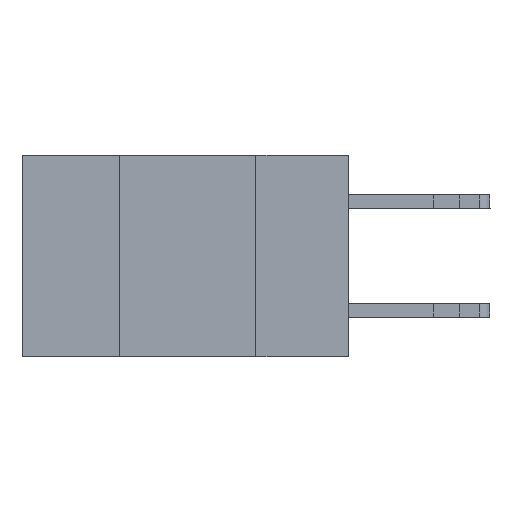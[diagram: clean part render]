
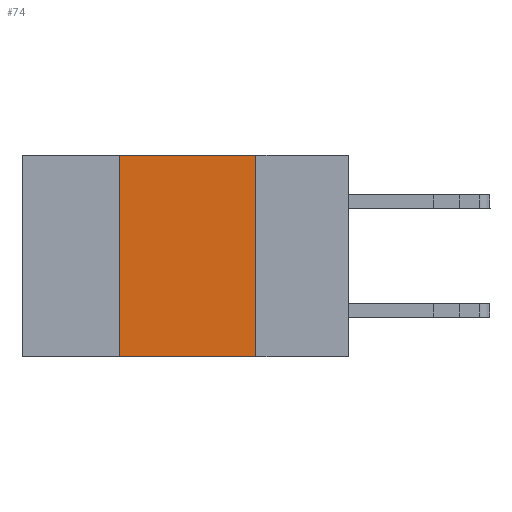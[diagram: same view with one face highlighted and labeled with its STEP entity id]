
A CAD part, left-side view. The second image highlights one B-rep face of the part: STEP entity #74.
In plain terms, the highlighted planar face has unit normal (-1, 0, 0).
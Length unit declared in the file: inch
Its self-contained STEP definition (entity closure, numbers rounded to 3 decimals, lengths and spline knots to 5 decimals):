
#74 = ADVANCED_FACE ( 'NONE', ( #4194 ), #6319, .F. ) ;
#379 = DIRECTION ( 'NONE',  ( 0., 0., -1. ) ) ;
#421 = DIRECTION ( 'NONE',  ( 0., 0., 1. ) ) ;
#565 = EDGE_CURVE ( 'NONE', #9878, #1397, #9668, .T. ) ;
#995 = AXIS2_PLACEMENT_3D ( 'NONE', #10096, #9133, #379 ) ;
#1397 = VERTEX_POINT ( 'NONE', #2305 ) ;
#1432 = EDGE_CURVE ( 'NONE', #7319, #1397, #5216, .T. ) ;
#1756 = LINE ( 'NONE', #9360, #6332 ) ;
#2246 = ORIENTED_EDGE ( 'NONE', *, *, #8146, .F. ) ;
#2305 = CARTESIAN_POINT ( 'NONE',  ( 0., 0.17, -0.37 ) ) ;
#3351 = LINE ( 'NONE', #12220, #3387 ) ;
#3387 = VECTOR ( 'NONE', #421, 39.37008 ) ;
#3593 = CARTESIAN_POINT ( 'NONE',  ( 0., 0.6, -0.37 ) ) ;
#3599 = DIRECTION ( 'NONE',  ( 0., -1., 0. ) ) ;
#3991 = ORIENTED_EDGE ( 'NONE', *, *, #565, .T. ) ;
#4194 = FACE_OUTER_BOUND ( 'NONE', #10234, .T. ) ;
#4781 = VERTEX_POINT ( 'NONE', #6317 ) ;
#5216 = LINE ( 'NONE', #11121, #9454 ) ;
#5626 = DIRECTION ( 'NONE',  ( 0., -1., 0. ) ) ;
#6211 = CARTESIAN_POINT ( 'NONE',  ( 0., 0.17, 0. ) ) ;
#6317 = CARTESIAN_POINT ( 'NONE',  ( 0., 0.42, 0. ) ) ;
#6319 = PLANE ( 'NONE',  #995 ) ;
#6332 = VECTOR ( 'NONE', #3599, 39.37008 ) ;
#7319 = VERTEX_POINT ( 'NONE', #6211 ) ;
#7679 = ORIENTED_EDGE ( 'NONE', *, *, #12114, .F. ) ;
#8146 = EDGE_CURVE ( 'NONE', #9878, #4781, #3351, .T. ) ;
#9133 = DIRECTION ( 'NONE',  ( 1., 0., 0. ) ) ;
#9360 = CARTESIAN_POINT ( 'NONE',  ( 0., 0.6, 0. ) ) ;
#9454 = VECTOR ( 'NONE', #12067, 39.37008 ) ;
#9668 = LINE ( 'NONE', #3593, #10858 ) ;
#9878 = VERTEX_POINT ( 'NONE', #10301 ) ;
#10096 = CARTESIAN_POINT ( 'NONE',  ( 0., 0.6, 0. ) ) ;
#10234 = EDGE_LOOP ( 'NONE', ( #11710, #7679, #2246, #3991 ) ) ;
#10301 = CARTESIAN_POINT ( 'NONE',  ( 0., 0.42, -0.37 ) ) ;
#10858 = VECTOR ( 'NONE', #5626, 39.37008 ) ;
#11121 = CARTESIAN_POINT ( 'NONE',  ( 0., 0.17, 0. ) ) ;
#11710 = ORIENTED_EDGE ( 'NONE', *, *, #1432, .F. ) ;
#12067 = DIRECTION ( 'NONE',  ( 0., 0., -1. ) ) ;
#12114 = EDGE_CURVE ( 'NONE', #4781, #7319, #1756, .T. ) ;
#12220 = CARTESIAN_POINT ( 'NONE',  ( 0., 0.42, 0. ) ) ;
